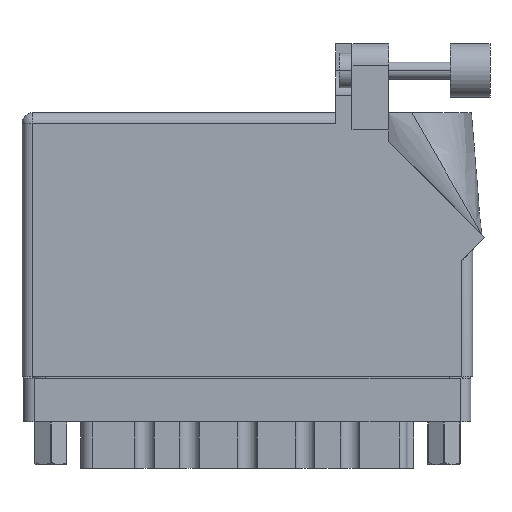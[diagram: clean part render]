
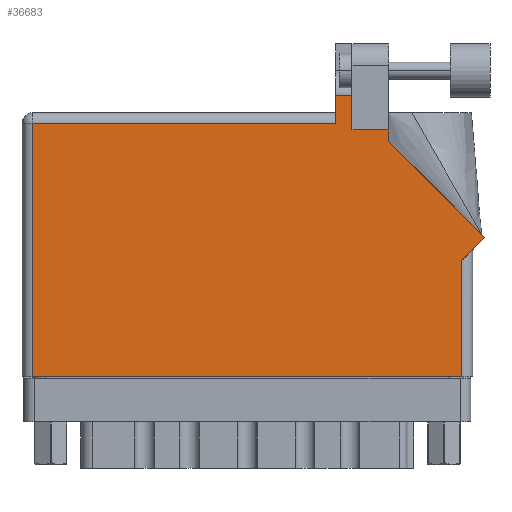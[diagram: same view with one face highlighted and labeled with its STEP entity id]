
A CAD part, front view. The second image highlights one B-rep face of the part: STEP entity #36683.
In plain terms, the highlighted face is planar.
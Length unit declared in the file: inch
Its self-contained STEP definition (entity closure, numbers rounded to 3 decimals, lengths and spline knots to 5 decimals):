
#81 = CARTESIAN_POINT ( 'NONE',  ( 2.24377, 1.6315, 0. ) ) ;
#1205 = PLANE ( 'NONE',  #33292 ) ;
#3027 = LINE ( 'NONE', #36288, #44668 ) ;
#3119 = ORIENTED_EDGE ( 'NONE', *, *, #42434, .T. ) ;
#3381 = DIRECTION ( 'NONE',  ( 0., 1., 0. ) ) ;
#4425 = VERTEX_POINT ( 'NONE', #58708 ) ;
#5793 = ORIENTED_EDGE ( 'NONE', *, *, #29385, .T. ) ;
#5929 = DIRECTION ( 'NONE',  ( -1., 0., 0. ) ) ;
#6190 = CARTESIAN_POINT ( 'NONE',  ( 1.819, 1.6315, 0. ) ) ;
#6300 = DIRECTION ( 'NONE',  ( 0., 1., 0. ) ) ;
#7493 = ORIENTED_EDGE ( 'NONE', *, *, #58405, .T. ) ;
#8656 = ORIENTED_EDGE ( 'NONE', *, *, #62569, .T. ) ;
#10771 = ORIENTED_EDGE ( 'NONE', *, *, #35389, .T. ) ;
#11327 = FACE_OUTER_BOUND ( 'NONE', #15148, .T. ) ;
#11452 = DIRECTION ( 'NONE',  ( 1., 0., 0. ) ) ;
#11722 = CARTESIAN_POINT ( 'NONE',  ( 1.913, 1.43, 0. ) ) ;
#12349 = VERTEX_POINT ( 'NONE', #36357 ) ;
#12505 = CARTESIAN_POINT ( 'NONE',  ( 1.819, 1.53, 0. ) ) ;
#14606 = VECTOR ( 'NONE', #52358, 39.37008 ) ;
#15148 = EDGE_LOOP ( 'NONE', ( #5793, #8656, #32790, #59925, #7493, #10771, #33083, #54638, #29190, #34047, #3119 ) ) ;
#15763 = CARTESIAN_POINT ( 'NONE',  ( 0., 1.53, 0. ) ) ;
#16580 = LINE ( 'NONE', #18203, #19645 ) ;
#16674 = LINE ( 'NONE', #12505, #34853 ) ;
#17850 = VECTOR ( 'NONE', #58711, 39.37008 ) ;
#18203 = CARTESIAN_POINT ( 'NONE',  ( 2.55, 0.737, 0. ) ) ;
#19645 = VECTOR ( 'NONE', #3381, 39.37008 ) ;
#20293 = VERTEX_POINT ( 'NONE', #27802 ) ;
#20453 = DIRECTION ( 'NONE',  ( -1., 0., 0. ) ) ;
#20656 = DIRECTION ( 'NONE',  ( -1., 0., 0. ) ) ;
#21407 = DIRECTION ( 'NONE',  ( 0., -1., 0. ) ) ;
#23004 = CARTESIAN_POINT ( 'NONE',  ( 2.612, 0.737, 0. ) ) ;
#24313 = EDGE_CURVE ( 'NONE', #50625, #55028, #16580, .T. ) ;
#24889 = CARTESIAN_POINT ( 'NONE',  ( 2.68271, 0.80771, 0. ) ) ;
#25165 = CARTESIAN_POINT ( 'NONE',  ( 1.913, 1.43, 0. ) ) ;
#27802 = CARTESIAN_POINT ( 'NONE',  ( 0.062, 0., 0. ) ) ;
#28574 = VECTOR ( 'NONE', #20453, 39.37008 ) ;
#29190 = ORIENTED_EDGE ( 'NONE', *, *, #44089, .T. ) ;
#29374 = LINE ( 'NONE', #39694, #28574 ) ;
#29385 = EDGE_CURVE ( 'NONE', #55410, #53295, #42519, .T. ) ;
#30592 = DIRECTION ( 'NONE',  ( 0., 1., 0. ) ) ;
#30922 = LINE ( 'NONE', #81, #51326 ) ;
#31623 = CARTESIAN_POINT ( 'NONE',  ( 1.819, 1.468, 0. ) ) ;
#31806 = EDGE_CURVE ( 'NONE', #55028, #51733, #37564, .T. ) ;
#32790 = ORIENTED_EDGE ( 'NONE', *, *, #35518, .T. ) ;
#33083 = ORIENTED_EDGE ( 'NONE', *, *, #24313, .T. ) ;
#33292 = AXIS2_PLACEMENT_3D ( 'NONE', #15763, #49661, #20656 ) ;
#34047 = ORIENTED_EDGE ( 'NONE', *, *, #36703, .T. ) ;
#34853 = VECTOR ( 'NONE', #21407, 39.37008 ) ;
#35389 = EDGE_CURVE ( 'NONE', #20293, #50625, #40890, .T. ) ;
#35518 = EDGE_CURVE ( 'NONE', #57153, #53533, #16674, .T. ) ;
#36288 = CARTESIAN_POINT ( 'NONE',  ( 2.126, 1.36442, 0. ) ) ;
#36357 = CARTESIAN_POINT ( 'NONE',  ( 2.126, 1.43, 0. ) ) ;
#36683 = ADVANCED_FACE ( 'NONE', ( #11327 ), #1205, .F. ) ;
#36703 = EDGE_CURVE ( 'NONE', #48378, #12349, #3027, .T. ) ;
#37334 = CARTESIAN_POINT ( 'NONE',  ( 0., 1.468, 0. ) ) ;
#37564 = LINE ( 'NONE', #23004, #48142 ) ;
#38231 = LINE ( 'NONE', #24889, #17850 ) ;
#38311 = CARTESIAN_POINT ( 'NONE',  ( 1.913, 1.6315, 0. ) ) ;
#38636 = VECTOR ( 'NONE', #54892, 39.37008 ) ;
#39677 = CARTESIAN_POINT ( 'NONE',  ( 0.062, 0., 0. ) ) ;
#39694 = CARTESIAN_POINT ( 'NONE',  ( 2.126, 1.43, 0. ) ) ;
#40059 = CARTESIAN_POINT ( 'NONE',  ( 0., 0., 0. ) ) ;
#40365 = CARTESIAN_POINT ( 'NONE',  ( 2.126, 1.36442, 0. ) ) ;
#40377 = CARTESIAN_POINT ( 'NONE',  ( 2.68271, 0.80771, 0. ) ) ;
#40890 = LINE ( 'NONE', #40059, #62039 ) ;
#42434 = EDGE_CURVE ( 'NONE', #12349, #55410, #29374, .T. ) ;
#42519 = LINE ( 'NONE', #25165, #54607 ) ;
#43086 = CARTESIAN_POINT ( 'NONE',  ( 2.55, 0.675, 0. ) ) ;
#44089 = EDGE_CURVE ( 'NONE', #51733, #48378, #38231, .T. ) ;
#44668 = VECTOR ( 'NONE', #30592, 39.37008 ) ;
#48142 = VECTOR ( 'NONE', #60844, 39.37008 ) ;
#48378 = VERTEX_POINT ( 'NONE', #40365 ) ;
#49661 = DIRECTION ( 'NONE',  ( 0., 0., -1. ) ) ;
#50625 = VERTEX_POINT ( 'NONE', #52411 ) ;
#51073 = EDGE_CURVE ( 'NONE', #53533, #4425, #52526, .T. ) ;
#51326 = VECTOR ( 'NONE', #5929, 39.37008 ) ;
#51733 = VERTEX_POINT ( 'NONE', #40377 ) ;
#52358 = DIRECTION ( 'NONE',  ( -1., 0., 0. ) ) ;
#52411 = CARTESIAN_POINT ( 'NONE',  ( 2.55, 0., 0. ) ) ;
#52526 = LINE ( 'NONE', #37334, #14606 ) ;
#53295 = VERTEX_POINT ( 'NONE', #38311 ) ;
#53533 = VERTEX_POINT ( 'NONE', #31623 ) ;
#54607 = VECTOR ( 'NONE', #6300, 39.37008 ) ;
#54638 = ORIENTED_EDGE ( 'NONE', *, *, #31806, .T. ) ;
#54892 = DIRECTION ( 'NONE',  ( 0., -1., 0. ) ) ;
#55028 = VERTEX_POINT ( 'NONE', #43086 ) ;
#55410 = VERTEX_POINT ( 'NONE', #11722 ) ;
#56120 = LINE ( 'NONE', #39677, #38636 ) ;
#57153 = VERTEX_POINT ( 'NONE', #6190 ) ;
#58405 = EDGE_CURVE ( 'NONE', #4425, #20293, #56120, .T. ) ;
#58708 = CARTESIAN_POINT ( 'NONE',  ( 0.062, 1.468, 0. ) ) ;
#58711 = DIRECTION ( 'NONE',  ( -0.707, 0.707, 0. ) ) ;
#59925 = ORIENTED_EDGE ( 'NONE', *, *, #51073, .T. ) ;
#60844 = DIRECTION ( 'NONE',  ( 0.707, 0.707, 0. ) ) ;
#62039 = VECTOR ( 'NONE', #11452, 39.37008 ) ;
#62569 = EDGE_CURVE ( 'NONE', #53295, #57153, #30922, .T. ) ;
